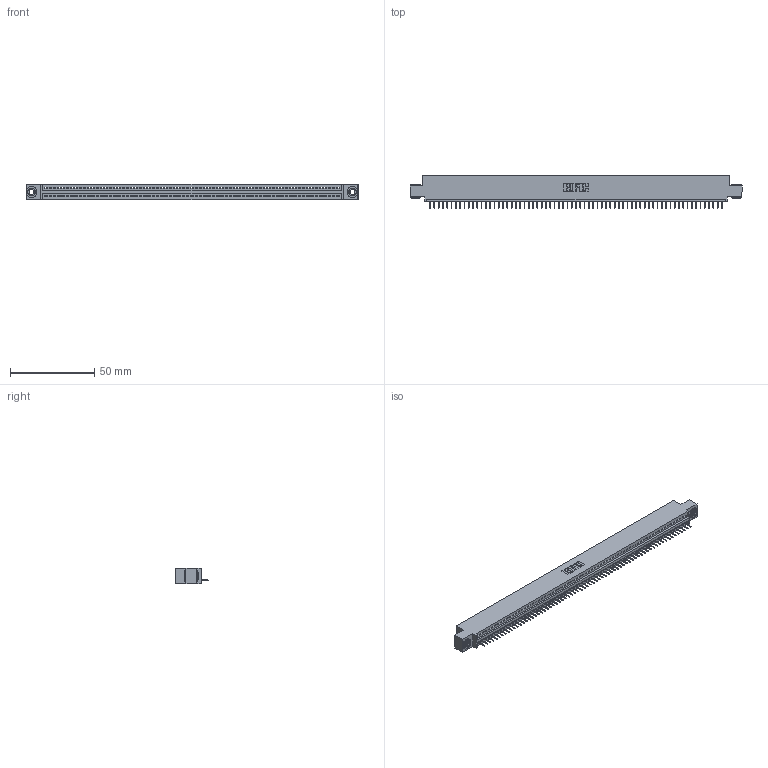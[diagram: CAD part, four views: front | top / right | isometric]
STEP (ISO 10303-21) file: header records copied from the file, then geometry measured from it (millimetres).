
FILE_DESCRIPTION (( 'STEP AP203' ), '1' );
FILE_NAME ('395-069-524-403.STEP', '2018-11-25T23:07:30', ( '' ), ( '' ), 'SwSTEP 2.0', 'SolidWorks 2016', '' );
FILE_SCHEMA (( 'CONFIG_CONTROL_DESIGN' ));
Length unit declared in the file: inch
Products named in the file (4): 345-250-002_345-250-002-102; 345 Part_0.110 Offset - 0.156 Dia-TH; 395-069-524-403; 345-292-001_345-293-124
Assembly tree (72 placements, depth 2):
  395-069-524-403
    345 Part_0.110 Offset - 0.156 Dia-TH
    345-292-001_345-293-124  x69
    345-250-002_345-250-002-102  x2
Bounding box: 196.47 x 19.35 x 9.4 mm (x, y, z)
Volume: 18555.5 mm3; surface area: 24450.3 mm2
Topology: 72 solids, 72 shells, 4446 faces, 12849 edges, 8286 vertices
Faces by surface type: plane 3268, cylinder 1170, cone 8
Entity records: 49152 total; most frequent: CARTESIAN_POINT 8490, ORIENTED_EDGE 8486, DIRECTION 7407, EDGE_CURVE 4243, VECTOR 3815, LINE 3815, VERTEX_POINT 2822, AXIS2_PLACEMENT_3D 1796
